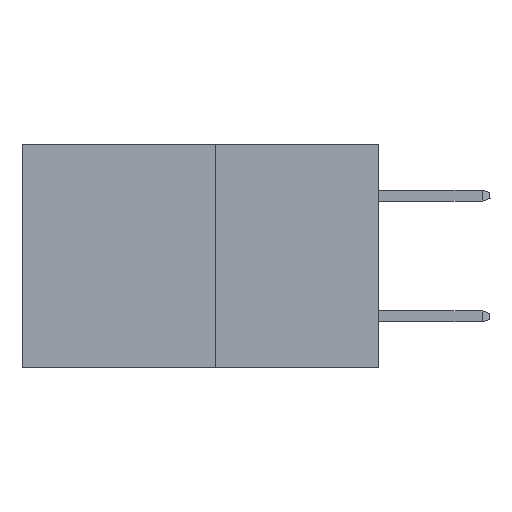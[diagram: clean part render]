
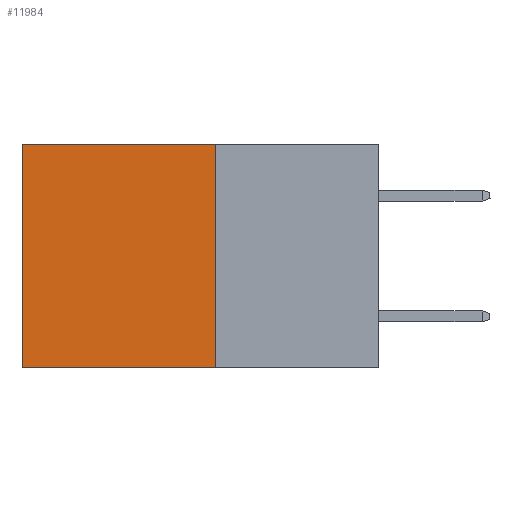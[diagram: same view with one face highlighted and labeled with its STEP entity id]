
A CAD part, left-side view. The second image highlights one B-rep face of the part: STEP entity #11984.
In plain terms, the highlighted planar face has unit normal (-1, 0, 0).
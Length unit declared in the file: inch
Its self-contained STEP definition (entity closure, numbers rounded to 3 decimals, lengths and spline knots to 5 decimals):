
#260 = DIRECTION ( 'NONE',  ( 0., 1., 0. ) ) ;
#1477 = VERTEX_POINT ( 'NONE', #28941 ) ;
#3017 = CARTESIAN_POINT ( 'NONE',  ( 0.277, 0.27, 0. ) ) ;
#4722 = CARTESIAN_POINT ( 'NONE',  ( 0.277, 0.27, -0.37 ) ) ;
#5247 = VERTEX_POINT ( 'NONE', #28230 ) ;
#8597 = VECTOR ( 'NONE', #260, 39.37008 ) ;
#9915 = VECTOR ( 'NONE', #29336, 39.37008 ) ;
#9951 = VERTEX_POINT ( 'NONE', #17593 ) ;
#10398 = DIRECTION ( 'NONE',  ( 0., 0., -1. ) ) ;
#11733 = CARTESIAN_POINT ( 'NONE',  ( 0.277, 0.27, -0.37 ) ) ;
#11984 = ADVANCED_FACE ( 'NONE', ( #29303 ), #28088, .F. ) ;
#12188 = ORIENTED_EDGE ( 'NONE', *, *, #31395, .F. ) ;
#13010 = ORIENTED_EDGE ( 'NONE', *, *, #27578, .T. ) ;
#13120 = VERTEX_POINT ( 'NONE', #19845 ) ;
#13655 = CARTESIAN_POINT ( 'NONE',  ( 0.277, 0.27, -0.37 ) ) ;
#13885 = VECTOR ( 'NONE', #30045, 39.37008 ) ;
#14456 = DIRECTION ( 'NONE',  ( 1., 0., 0. ) ) ;
#15010 = EDGE_CURVE ( 'NONE', #1477, #13120, #32111, .T. ) ;
#15892 = EDGE_LOOP ( 'NONE', ( #30365, #12188, #22577, #13010 ) ) ;
#17159 = LINE ( 'NONE', #4722, #9915 ) ;
#17593 = CARTESIAN_POINT ( 'NONE',  ( 0.277, 0.27, 0. ) ) ;
#19845 = CARTESIAN_POINT ( 'NONE',  ( 0.277, 0.59, -0.37 ) ) ;
#21331 = AXIS2_PLACEMENT_3D ( 'NONE', #11733, #14456, #33583 ) ;
#22577 = ORIENTED_EDGE ( 'NONE', *, *, #27294, .F. ) ;
#25676 = VECTOR ( 'NONE', #10398, 39.37008 ) ;
#26731 = CARTESIAN_POINT ( 'NONE',  ( 0.277, 0.59, -0.37 ) ) ;
#27294 = EDGE_CURVE ( 'NONE', #9951, #5247, #17159, .T. ) ;
#27578 = EDGE_CURVE ( 'NONE', #9951, #1477, #30409, .T. ) ;
#28088 = PLANE ( 'NONE',  #21331 ) ;
#28230 = CARTESIAN_POINT ( 'NONE',  ( 0.277, 0.27, -0.37 ) ) ;
#28426 = LINE ( 'NONE', #13655, #13885 ) ;
#28941 = CARTESIAN_POINT ( 'NONE',  ( 0.277, 0.59, 0. ) ) ;
#29303 = FACE_OUTER_BOUND ( 'NONE', #15892, .T. ) ;
#29336 = DIRECTION ( 'NONE',  ( 0., 0., -1. ) ) ;
#30045 = DIRECTION ( 'NONE',  ( 0., 1., 0. ) ) ;
#30365 = ORIENTED_EDGE ( 'NONE', *, *, #15010, .T. ) ;
#30409 = LINE ( 'NONE', #3017, #8597 ) ;
#31395 = EDGE_CURVE ( 'NONE', #5247, #13120, #28426, .T. ) ;
#32111 = LINE ( 'NONE', #26731, #25676 ) ;
#33583 = DIRECTION ( 'NONE',  ( 0., 0., -1. ) ) ;
